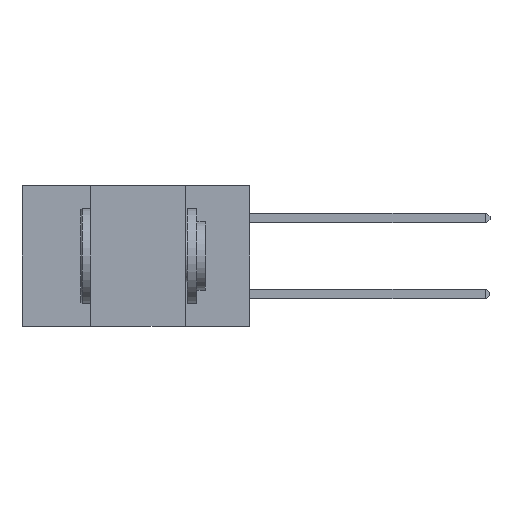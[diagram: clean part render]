
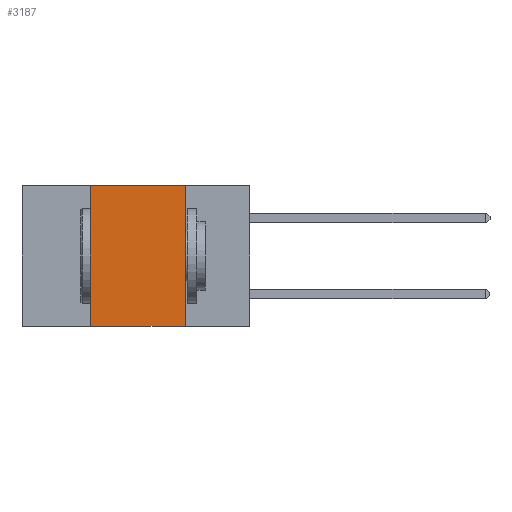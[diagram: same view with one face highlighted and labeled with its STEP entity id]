
A CAD part, left-side view. The second image highlights one B-rep face of the part: STEP entity #3187.
In plain terms, the highlighted planar face has unit normal (-1, 0, 0).
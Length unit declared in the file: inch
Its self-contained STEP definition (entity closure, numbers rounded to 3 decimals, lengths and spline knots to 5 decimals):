
#570 = EDGE_CURVE ( 'NONE', #14368, #13245, #10308, .T. ) ;
#714 = ORIENTED_EDGE ( 'NONE', *, *, #12936, .F. ) ;
#1979 = LINE ( 'NONE', #9953, #11443 ) ;
#2089 = VERTEX_POINT ( 'NONE', #8372 ) ;
#3187 = ADVANCED_FACE ( 'NONE', ( #9225 ), #11385, .F. ) ;
#3211 = CARTESIAN_POINT ( 'NONE',  ( 0., 0.17, -0.37 ) ) ;
#4306 = CARTESIAN_POINT ( 'NONE',  ( 0., 0.6, -0.37 ) ) ;
#4694 = VECTOR ( 'NONE', #14511, 39.37008 ) ;
#5019 = EDGE_CURVE ( 'NONE', #2089, #13245, #8540, .T. ) ;
#5489 = EDGE_LOOP ( 'NONE', ( #9565, #714, #12322, #8287 ) ) ;
#5509 = EDGE_CURVE ( 'NONE', #14368, #6793, #1979, .T. ) ;
#6401 = CARTESIAN_POINT ( 'NONE',  ( 0., 0.6, 0. ) ) ;
#6793 = VERTEX_POINT ( 'NONE', #14216 ) ;
#6857 = CARTESIAN_POINT ( 'NONE',  ( 0., 0.42, -0.37 ) ) ;
#6871 = VECTOR ( 'NONE', #14347, 39.37008 ) ;
#7574 = LINE ( 'NONE', #6401, #13648 ) ;
#8287 = ORIENTED_EDGE ( 'NONE', *, *, #570, .T. ) ;
#8372 = CARTESIAN_POINT ( 'NONE',  ( 0., 0.17, 0. ) ) ;
#8540 = LINE ( 'NONE', #14611, #4694 ) ;
#8934 = DIRECTION ( 'NONE',  ( 0., -1., 0. ) ) ;
#9225 = FACE_OUTER_BOUND ( 'NONE', #5489, .T. ) ;
#9565 = ORIENTED_EDGE ( 'NONE', *, *, #5019, .F. ) ;
#9899 = DIRECTION ( 'NONE',  ( 0., 0., 1. ) ) ;
#9953 = CARTESIAN_POINT ( 'NONE',  ( 0., 0.42, 0. ) ) ;
#10308 = LINE ( 'NONE', #4306, #6871 ) ;
#10972 = DIRECTION ( 'NONE',  ( 0., 0., -1. ) ) ;
#11071 = DIRECTION ( 'NONE',  ( 1., 0., 0. ) ) ;
#11080 = CARTESIAN_POINT ( 'NONE',  ( 0., 0.6, 0. ) ) ;
#11385 = PLANE ( 'NONE',  #15159 ) ;
#11443 = VECTOR ( 'NONE', #9899, 39.37008 ) ;
#12322 = ORIENTED_EDGE ( 'NONE', *, *, #5509, .F. ) ;
#12936 = EDGE_CURVE ( 'NONE', #6793, #2089, #7574, .T. ) ;
#13245 = VERTEX_POINT ( 'NONE', #3211 ) ;
#13648 = VECTOR ( 'NONE', #8934, 39.37008 ) ;
#14216 = CARTESIAN_POINT ( 'NONE',  ( 0., 0.42, 0. ) ) ;
#14347 = DIRECTION ( 'NONE',  ( 0., -1., 0. ) ) ;
#14368 = VERTEX_POINT ( 'NONE', #6857 ) ;
#14511 = DIRECTION ( 'NONE',  ( 0., 0., -1. ) ) ;
#14611 = CARTESIAN_POINT ( 'NONE',  ( 0., 0.17, 0. ) ) ;
#15159 = AXIS2_PLACEMENT_3D ( 'NONE', #11080, #11071, #10972 ) ;
